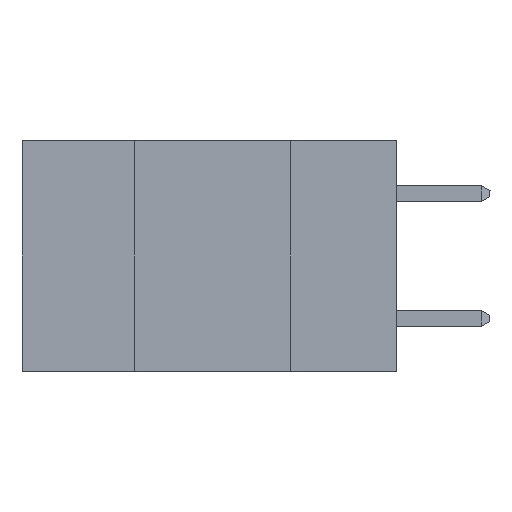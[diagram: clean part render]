
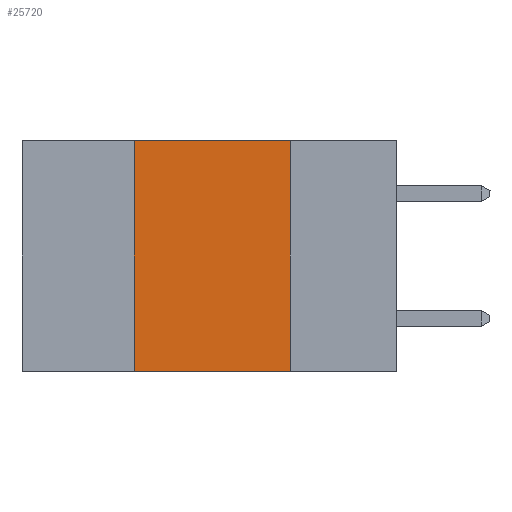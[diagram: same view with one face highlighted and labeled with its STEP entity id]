
A CAD part, left-side view. The second image highlights one B-rep face of the part: STEP entity #25720.
In plain terms, the highlighted planar face has unit normal (-1, 0, 0).
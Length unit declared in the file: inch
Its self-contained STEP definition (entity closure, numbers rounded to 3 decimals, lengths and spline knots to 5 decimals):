
#986 = EDGE_CURVE ( 'NONE', #18190, #20601, #10572, .T. ) ;
#2209 = DIRECTION ( 'NONE',  ( 0., 0., 1. ) ) ;
#2440 = CARTESIAN_POINT ( 'NONE',  ( 0., 0.6, 0. ) ) ;
#2661 = CARTESIAN_POINT ( 'NONE',  ( 0., 0.17, 0. ) ) ;
#2844 = VECTOR ( 'NONE', #2209, 39.37008 ) ;
#3041 = VECTOR ( 'NONE', #13285, 39.37008 ) ;
#4315 = CARTESIAN_POINT ( 'NONE',  ( 0., 0.6, 0. ) ) ;
#4397 = EDGE_CURVE ( 'NONE', #7533, #20601, #25034, .T. ) ;
#5844 = AXIS2_PLACEMENT_3D ( 'NONE', #4315, #6458, #21365 ) ;
#6127 = DIRECTION ( 'NONE',  ( 0., -1., 0. ) ) ;
#6458 = DIRECTION ( 'NONE',  ( 1., 0., 0. ) ) ;
#6718 = EDGE_CURVE ( 'NONE', #18190, #19220, #24850, .T. ) ;
#7533 = VERTEX_POINT ( 'NONE', #11214 ) ;
#7962 = ORIENTED_EDGE ( 'NONE', *, *, #986, .T. ) ;
#8448 = CARTESIAN_POINT ( 'NONE',  ( 0., 0.42, 0. ) ) ;
#10572 = LINE ( 'NONE', #13305, #26885 ) ;
#11214 = CARTESIAN_POINT ( 'NONE',  ( 0., 0.17, 0. ) ) ;
#12054 = VECTOR ( 'NONE', #17338, 39.37008 ) ;
#12321 = ORIENTED_EDGE ( 'NONE', *, *, #4397, .F. ) ;
#12711 = LINE ( 'NONE', #2440, #12054 ) ;
#12718 = FACE_OUTER_BOUND ( 'NONE', #24828, .T. ) ;
#12787 = PLANE ( 'NONE',  #5844 ) ;
#12846 = CARTESIAN_POINT ( 'NONE',  ( 0., 0.42, 0. ) ) ;
#13285 = DIRECTION ( 'NONE',  ( 0., 0., -1. ) ) ;
#13305 = CARTESIAN_POINT ( 'NONE',  ( 0., 0.6, -0.37 ) ) ;
#15520 = EDGE_CURVE ( 'NONE', #19220, #7533, #12711, .T. ) ;
#17338 = DIRECTION ( 'NONE',  ( 0., -1., 0. ) ) ;
#18190 = VERTEX_POINT ( 'NONE', #24503 ) ;
#19220 = VERTEX_POINT ( 'NONE', #8448 ) ;
#20199 = ORIENTED_EDGE ( 'NONE', *, *, #15520, .F. ) ;
#20601 = VERTEX_POINT ( 'NONE', #22037 ) ;
#21365 = DIRECTION ( 'NONE',  ( 0., 0., -1. ) ) ;
#21872 = ORIENTED_EDGE ( 'NONE', *, *, #6718, .F. ) ;
#22037 = CARTESIAN_POINT ( 'NONE',  ( 0., 0.17, -0.37 ) ) ;
#24503 = CARTESIAN_POINT ( 'NONE',  ( 0., 0.42, -0.37 ) ) ;
#24828 = EDGE_LOOP ( 'NONE', ( #12321, #20199, #21872, #7962 ) ) ;
#24850 = LINE ( 'NONE', #12846, #2844 ) ;
#25034 = LINE ( 'NONE', #2661, #3041 ) ;
#25720 = ADVANCED_FACE ( 'NONE', ( #12718 ), #12787, .F. ) ;
#26885 = VECTOR ( 'NONE', #6127, 39.37008 ) ;
